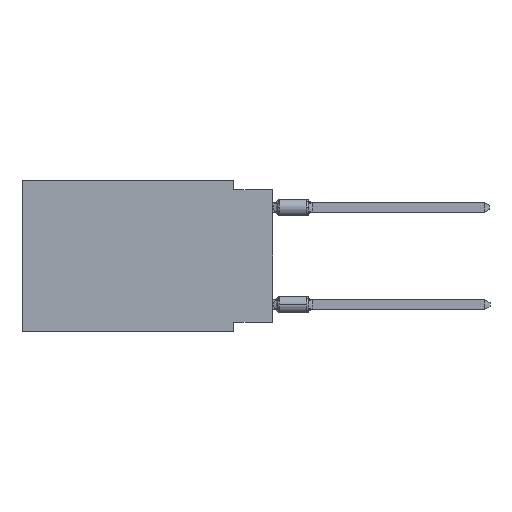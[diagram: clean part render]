
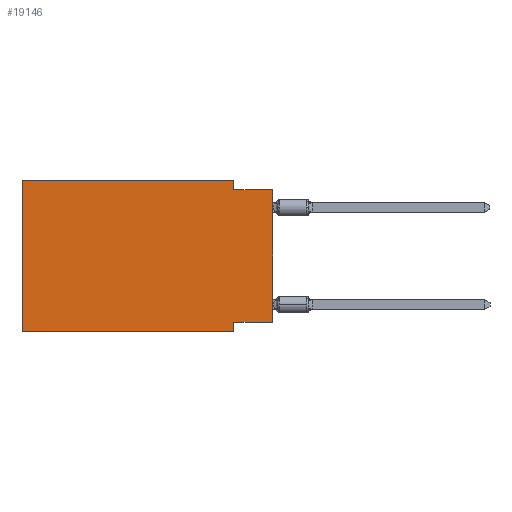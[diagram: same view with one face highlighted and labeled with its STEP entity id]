
A CAD part, left-side view. The second image highlights one B-rep face of the part: STEP entity #19146.
In plain terms, the highlighted planar face has unit normal (-1, 0, 0).
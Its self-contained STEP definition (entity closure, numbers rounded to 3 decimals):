
#1114 = CARTESIAN_POINT ( 'NONE',  ( 0., 16.383, 0. ) ) ;
#1861 = DIRECTION ( 'NONE',  ( 0., 0., -1. ) ) ;
#2674 = ORIENTED_EDGE ( 'NONE', *, *, #4901, .F. ) ;
#2714 = DIRECTION ( 'NONE',  ( 0., 0., 1. ) ) ;
#2799 = CARTESIAN_POINT ( 'NONE',  ( 0., 2.54, -9.906 ) ) ;
#2899 = VERTEX_POINT ( 'NONE', #20684 ) ;
#3321 = CARTESIAN_POINT ( 'NONE',  ( 0., 2.54, -9.271 ) ) ;
#3570 = EDGE_CURVE ( 'NONE', #8618, #14348, #12796, .T. ) ;
#4097 = VECTOR ( 'NONE', #10946, 1000. ) ;
#4518 = VECTOR ( 'NONE', #1861, 1000. ) ;
#4733 = LINE ( 'NONE', #19051, #10186 ) ;
#4901 = EDGE_CURVE ( 'NONE', #2899, #7924, #6515, .T. ) ;
#5257 = AXIS2_PLACEMENT_3D ( 'NONE', #18189, #10721, #8888 ) ;
#5328 = CARTESIAN_POINT ( 'NONE',  ( 0., 2.54, -0.635 ) ) ;
#5444 = LINE ( 'NONE', #11435, #4097 ) ;
#6182 = ORIENTED_EDGE ( 'NONE', *, *, #10062, .F. ) ;
#6515 = LINE ( 'NONE', #19469, #18104 ) ;
#6761 = DIRECTION ( 'NONE',  ( 0., -1., 0. ) ) ;
#7924 = VERTEX_POINT ( 'NONE', #22062 ) ;
#8410 = VERTEX_POINT ( 'NONE', #2799 ) ;
#8618 = VERTEX_POINT ( 'NONE', #12563 ) ;
#8888 = DIRECTION ( 'NONE',  ( 0., 0., -1. ) ) ;
#9063 = DIRECTION ( 'NONE',  ( 0., -1., 0. ) ) ;
#9192 = CARTESIAN_POINT ( 'NONE',  ( 0., 16.383, -9.906 ) ) ;
#9550 = LINE ( 'NONE', #9192, #16961 ) ;
#9571 = LINE ( 'NONE', #17048, #4518 ) ;
#10062 = EDGE_CURVE ( 'NONE', #20611, #12273, #4733, .T. ) ;
#10186 = VECTOR ( 'NONE', #13537, 1000. ) ;
#10566 = EDGE_CURVE ( 'NONE', #7924, #20611, #20991, .T. ) ;
#10613 = DIRECTION ( 'NONE',  ( 0., 1., 0. ) ) ;
#10721 = DIRECTION ( 'NONE',  ( 1., 0., 0. ) ) ;
#10946 = DIRECTION ( 'NONE',  ( 0., -1., 0. ) ) ;
#11435 = CARTESIAN_POINT ( 'NONE',  ( 0., 0., -0.635 ) ) ;
#12273 = VERTEX_POINT ( 'NONE', #5328 ) ;
#12431 = EDGE_CURVE ( 'NONE', #12273, #13130, #5444, .T. ) ;
#12557 = PLANE ( 'NONE',  #5257 ) ;
#12563 = CARTESIAN_POINT ( 'NONE',  ( 0., 0., -9.271 ) ) ;
#12566 = CARTESIAN_POINT ( 'NONE',  ( 0., 0., -9.271 ) ) ;
#12705 = LINE ( 'NONE', #16382, #23020 ) ;
#12796 = LINE ( 'NONE', #12566, #22333 ) ;
#13130 = VERTEX_POINT ( 'NONE', #24057 ) ;
#13517 = ORIENTED_EDGE ( 'NONE', *, *, #12431, .F. ) ;
#13537 = DIRECTION ( 'NONE',  ( 0., 0., -1. ) ) ;
#14028 = EDGE_LOOP ( 'NONE', ( #21154, #13517, #6182, #17700, #2674, #23306, #19664, #17708 ) ) ;
#14348 = VERTEX_POINT ( 'NONE', #3321 ) ;
#14482 = EDGE_CURVE ( 'NONE', #2899, #8410, #9550, .T. ) ;
#14824 = EDGE_CURVE ( 'NONE', #8618, #13130, #12705, .T. ) ;
#16382 = CARTESIAN_POINT ( 'NONE',  ( 0., 0., 0. ) ) ;
#16961 = VECTOR ( 'NONE', #9063, 1000. ) ;
#17048 = CARTESIAN_POINT ( 'NONE',  ( 0., 2.54, -9.906 ) ) ;
#17134 = VECTOR ( 'NONE', #6761, 1000. ) ;
#17700 = ORIENTED_EDGE ( 'NONE', *, *, #10566, .F. ) ;
#17708 = ORIENTED_EDGE ( 'NONE', *, *, #3570, .F. ) ;
#18104 = VECTOR ( 'NONE', #2714, 1000. ) ;
#18189 = CARTESIAN_POINT ( 'NONE',  ( 0., 16.383, 0. ) ) ;
#19051 = CARTESIAN_POINT ( 'NONE',  ( 0., 2.54, 0. ) ) ;
#19146 = ADVANCED_FACE ( 'NONE', ( #23683 ), #12557, .F. ) ;
#19277 = CARTESIAN_POINT ( 'NONE',  ( 0., 2.54, 0. ) ) ;
#19469 = CARTESIAN_POINT ( 'NONE',  ( 0., 16.383, 0. ) ) ;
#19664 = ORIENTED_EDGE ( 'NONE', *, *, #23301, .F. ) ;
#20611 = VERTEX_POINT ( 'NONE', #19277 ) ;
#20684 = CARTESIAN_POINT ( 'NONE',  ( 0., 16.383, -9.906 ) ) ;
#20991 = LINE ( 'NONE', #1114, #17134 ) ;
#21154 = ORIENTED_EDGE ( 'NONE', *, *, #14824, .T. ) ;
#22062 = CARTESIAN_POINT ( 'NONE',  ( 0., 16.383, 0. ) ) ;
#22333 = VECTOR ( 'NONE', #10613, 1000. ) ;
#23020 = VECTOR ( 'NONE', #23816, 1000. ) ;
#23301 = EDGE_CURVE ( 'NONE', #14348, #8410, #9571, .T. ) ;
#23306 = ORIENTED_EDGE ( 'NONE', *, *, #14482, .T. ) ;
#23683 = FACE_OUTER_BOUND ( 'NONE', #14028, .T. ) ;
#23816 = DIRECTION ( 'NONE',  ( 0., 0., 1. ) ) ;
#24057 = CARTESIAN_POINT ( 'NONE',  ( 0., 0., -0.635 ) ) ;
